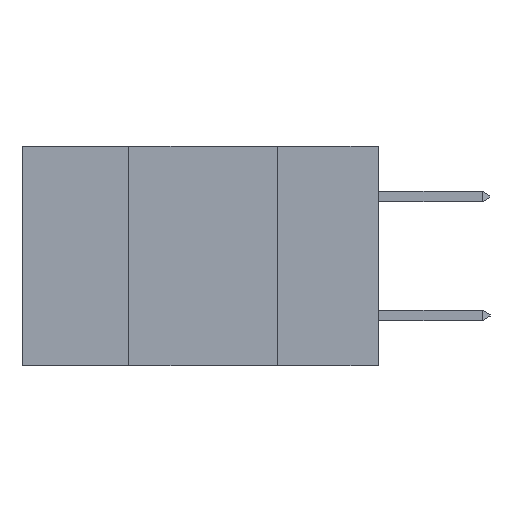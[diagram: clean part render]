
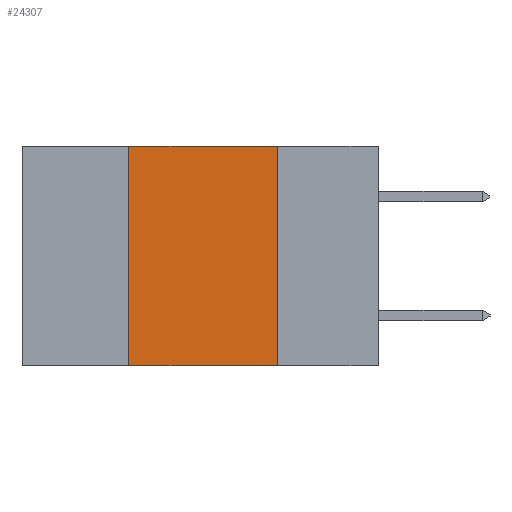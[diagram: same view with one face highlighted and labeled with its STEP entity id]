
A CAD part, left-side view. The second image highlights one B-rep face of the part: STEP entity #24307.
In plain terms, the highlighted planar face has unit normal (-1, 0, 0).
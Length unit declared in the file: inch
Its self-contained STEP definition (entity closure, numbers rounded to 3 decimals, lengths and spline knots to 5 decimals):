
#99 = EDGE_CURVE ( 'NONE', #13261, #6273, #16219, .T. ) ;
#416 = AXIS2_PLACEMENT_3D ( 'NONE', #11155, #7260, #20652 ) ;
#1384 = VERTEX_POINT ( 'NONE', #6771 ) ;
#2041 = DIRECTION ( 'NONE',  ( 0., 0., -1. ) ) ;
#2666 = ORIENTED_EDGE ( 'NONE', *, *, #17718, .T. ) ;
#3365 = PLANE ( 'NONE',  #416 ) ;
#4009 = CARTESIAN_POINT ( 'NONE',  ( 0., 0.17, -0.37 ) ) ;
#4376 = LINE ( 'NONE', #4009, #22879 ) ;
#5408 = CARTESIAN_POINT ( 'NONE',  ( 0., 0.42, -0.37 ) ) ;
#6273 = VERTEX_POINT ( 'NONE', #17863 ) ;
#6771 = CARTESIAN_POINT ( 'NONE',  ( 0., 0.17, -0.37 ) ) ;
#7120 = ORIENTED_EDGE ( 'NONE', *, *, #22259, .F. ) ;
#7260 = DIRECTION ( 'NONE',  ( 1., 0., 0. ) ) ;
#8612 = VECTOR ( 'NONE', #16389, 39.37008 ) ;
#9235 = CARTESIAN_POINT ( 'NONE',  ( 0., 0.42, -0.37 ) ) ;
#9238 = LINE ( 'NONE', #23813, #8612 ) ;
#11115 = CARTESIAN_POINT ( 'NONE',  ( 0., 0.17, 0. ) ) ;
#11155 = CARTESIAN_POINT ( 'NONE',  ( 0., 0.6, 0. ) ) ;
#11721 = ORIENTED_EDGE ( 'NONE', *, *, #99, .F. ) ;
#12701 = VECTOR ( 'NONE', #14689, 39.37008 ) ;
#13261 = VERTEX_POINT ( 'NONE', #5408 ) ;
#13646 = ORIENTED_EDGE ( 'NONE', *, *, #13988, .F. ) ;
#13663 = EDGE_LOOP ( 'NONE', ( #13646, #7120, #11721, #2666 ) ) ;
#13988 = EDGE_CURVE ( 'NONE', #15716, #1384, #4376, .T. ) ;
#14689 = DIRECTION ( 'NONE',  ( 0., -1., 0. ) ) ;
#15289 = FACE_OUTER_BOUND ( 'NONE', #13663, .T. ) ;
#15612 = VECTOR ( 'NONE', #20783, 39.37008 ) ;
#15716 = VERTEX_POINT ( 'NONE', #11115 ) ;
#16219 = LINE ( 'NONE', #9235, #15612 ) ;
#16389 = DIRECTION ( 'NONE',  ( 0., -1., 0. ) ) ;
#17716 = LINE ( 'NONE', #18460, #12701 ) ;
#17718 = EDGE_CURVE ( 'NONE', #13261, #1384, #17716, .T. ) ;
#17863 = CARTESIAN_POINT ( 'NONE',  ( 0., 0.42, 0. ) ) ;
#18460 = CARTESIAN_POINT ( 'NONE',  ( 0., 0.6, -0.37 ) ) ;
#20652 = DIRECTION ( 'NONE',  ( 0., 0., -1. ) ) ;
#20783 = DIRECTION ( 'NONE',  ( 0., 0., 1. ) ) ;
#22259 = EDGE_CURVE ( 'NONE', #6273, #15716, #9238, .T. ) ;
#22879 = VECTOR ( 'NONE', #2041, 39.37008 ) ;
#23813 = CARTESIAN_POINT ( 'NONE',  ( 0., 0.6, 0. ) ) ;
#24307 = ADVANCED_FACE ( 'NONE', ( #15289 ), #3365, .F. ) ;
